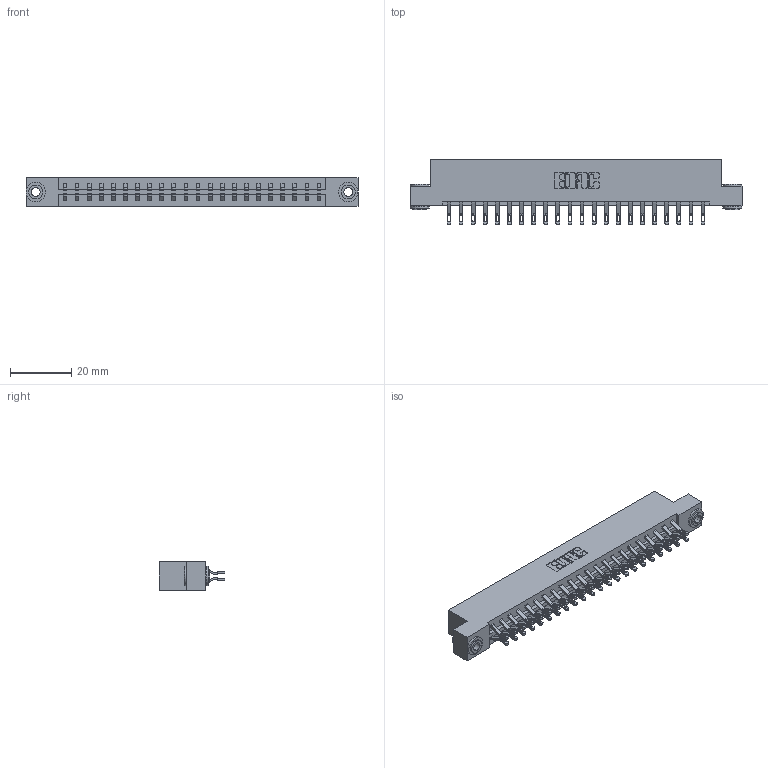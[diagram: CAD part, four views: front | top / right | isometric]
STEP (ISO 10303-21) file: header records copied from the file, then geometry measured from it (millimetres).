
FILE_DESCRIPTION (( 'STEP AP203' ), '1' );
FILE_NAME ('833-044-555-203.STEP', '2020-06-04T01:43:53', ( '' ), ( '' ), 'SwSTEP 2.0', 'SolidWorks 2020', '' );
FILE_SCHEMA (( 'CONFIG_CONTROL_DESIGN' ));
Length unit declared in the file: inch
Products named in the file (4): 345-250-002_345-250-002-102; 833-044-555-203; 345-292-001_555 Tail; 833 Part_Flush - .156 Dia - TH
Assembly tree (47 placements, depth 2):
  833-044-555-203
    833 Part_Flush - .156 Dia - TH
    345-292-001_555 Tail  x44
    345-250-002_345-250-002-102  x2
Bounding box: 108.71 x 21.47 x 9.4 mm (x, y, z)
Volume: 11058.9 mm3; surface area: 13557.6 mm2
Topology: 47 solids, 47 shells, 2704 faces, 8439 edges, 5622 vertices
Faces by surface type: plane 1576, cylinder 1120, cone 8
Entity records: 17716 total; most frequent: CARTESIAN_POINT 2971, ORIENTED_EDGE 2870, DIRECTION 2577, EDGE_CURVE 1435, LINE 1263, VECTOR 1263, VERTEX_POINT 954, AXIS2_PLACEMENT_3D 657
